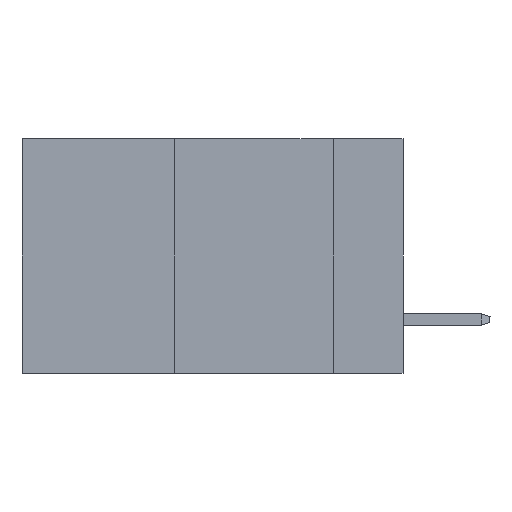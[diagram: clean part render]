
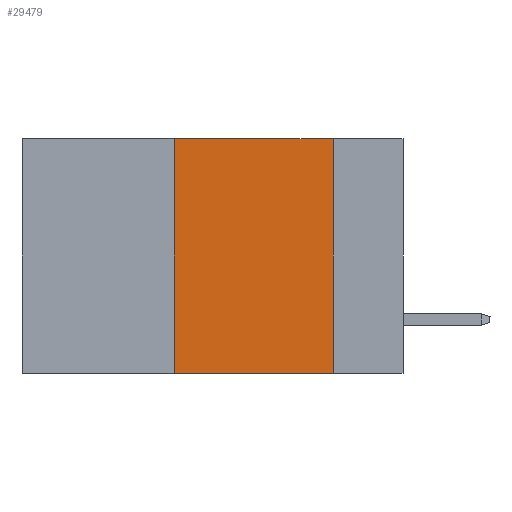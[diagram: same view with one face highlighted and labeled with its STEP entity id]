
A CAD part, left-side view. The second image highlights one B-rep face of the part: STEP entity #29479.
In plain terms, the highlighted planar face has unit normal (-1, 0, 0).
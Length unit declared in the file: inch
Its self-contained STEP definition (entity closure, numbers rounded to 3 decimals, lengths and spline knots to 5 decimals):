
#366 = CARTESIAN_POINT ( 'NONE',  ( 0., 0.11, -0.37 ) ) ;
#2639 = PLANE ( 'NONE',  #18286 ) ;
#2935 = ORIENTED_EDGE ( 'NONE', *, *, #6267, .F. ) ;
#3676 = ORIENTED_EDGE ( 'NONE', *, *, #14835, .F. ) ;
#4063 = LINE ( 'NONE', #13967, #19026 ) ;
#5193 = DIRECTION ( 'NONE',  ( 0., -1., 0. ) ) ;
#6267 = EDGE_CURVE ( 'NONE', #10116, #39268, #21841, .T. ) ;
#7336 = EDGE_LOOP ( 'NONE', ( #3676, #2935, #36680, #7942 ) ) ;
#7942 = ORIENTED_EDGE ( 'NONE', *, *, #12710, .T. ) ;
#9079 = CARTESIAN_POINT ( 'NONE',  ( 0., 0.36, 0. ) ) ;
#10116 = VERTEX_POINT ( 'NONE', #16979 ) ;
#12136 = DIRECTION ( 'NONE',  ( 1., 0., 0. ) ) ;
#12465 = DIRECTION ( 'NONE',  ( 0., 0., 1. ) ) ;
#12710 = EDGE_CURVE ( 'NONE', #24788, #28804, #24298, .T. ) ;
#13533 = CARTESIAN_POINT ( 'NONE',  ( 0., 0.11, 0. ) ) ;
#13967 = CARTESIAN_POINT ( 'NONE',  ( 0., 0.11, 0. ) ) ;
#14835 = EDGE_CURVE ( 'NONE', #39268, #28804, #4063, .T. ) ;
#16231 = VECTOR ( 'NONE', #37157, 39.37008 ) ;
#16979 = CARTESIAN_POINT ( 'NONE',  ( 0., 0.36, 0. ) ) ;
#18286 = AXIS2_PLACEMENT_3D ( 'NONE', #24377, #12136, #25215 ) ;
#18680 = CARTESIAN_POINT ( 'NONE',  ( 0., 0.6, 0. ) ) ;
#19026 = VECTOR ( 'NONE', #26826, 39.37008 ) ;
#21319 = CARTESIAN_POINT ( 'NONE',  ( 0., 0.6, -0.37 ) ) ;
#21841 = LINE ( 'NONE', #18680, #27157 ) ;
#24298 = LINE ( 'NONE', #21319, #16231 ) ;
#24377 = CARTESIAN_POINT ( 'NONE',  ( 0., 0.6, 0. ) ) ;
#24788 = VERTEX_POINT ( 'NONE', #39875 ) ;
#24912 = LINE ( 'NONE', #9079, #25417 ) ;
#25215 = DIRECTION ( 'NONE',  ( 0., 0., -1. ) ) ;
#25417 = VECTOR ( 'NONE', #12465, 39.37008 ) ;
#26826 = DIRECTION ( 'NONE',  ( 0., 0., -1. ) ) ;
#27157 = VECTOR ( 'NONE', #5193, 39.37008 ) ;
#28804 = VERTEX_POINT ( 'NONE', #366 ) ;
#29479 = ADVANCED_FACE ( 'NONE', ( #31137 ), #2639, .F. ) ;
#31137 = FACE_OUTER_BOUND ( 'NONE', #7336, .T. ) ;
#36680 = ORIENTED_EDGE ( 'NONE', *, *, #38553, .F. ) ;
#37157 = DIRECTION ( 'NONE',  ( 0., -1., 0. ) ) ;
#38553 = EDGE_CURVE ( 'NONE', #24788, #10116, #24912, .T. ) ;
#39268 = VERTEX_POINT ( 'NONE', #13533 ) ;
#39875 = CARTESIAN_POINT ( 'NONE',  ( 0., 0.36, -0.37 ) ) ;
